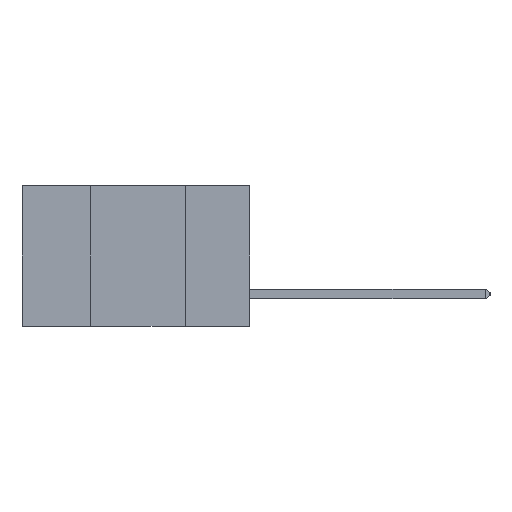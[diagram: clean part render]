
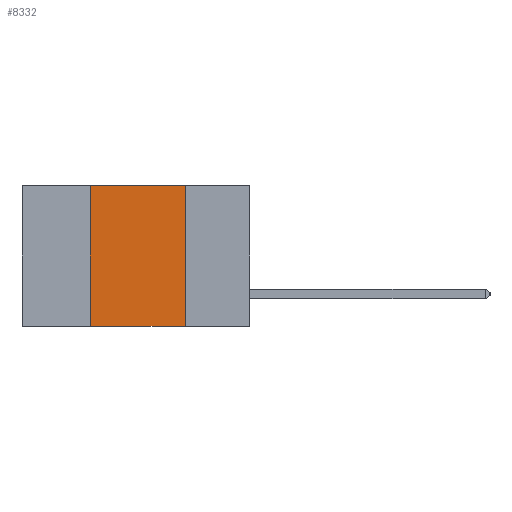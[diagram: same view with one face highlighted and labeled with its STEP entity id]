
A CAD part, left-side view. The second image highlights one B-rep face of the part: STEP entity #8332.
In plain terms, the highlighted planar face has unit normal (-1, 0, 0).
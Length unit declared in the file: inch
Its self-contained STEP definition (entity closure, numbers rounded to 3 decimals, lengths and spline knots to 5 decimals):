
#283 = VERTEX_POINT ( 'NONE', #540 ) ;
#540 = CARTESIAN_POINT ( 'NONE',  ( 0., 0.42, 0. ) ) ;
#607 = PLANE ( 'NONE',  #7331 ) ;
#1368 = ORIENTED_EDGE ( 'NONE', *, *, #8800, .T. ) ;
#1800 = CARTESIAN_POINT ( 'NONE',  ( 0., 0.6, 0. ) ) ;
#1893 = DIRECTION ( 'NONE',  ( 0., 0., 1. ) ) ;
#2639 = VECTOR ( 'NONE', #13578, 39.37008 ) ;
#3047 = LINE ( 'NONE', #1800, #2639 ) ;
#3228 = DIRECTION ( 'NONE',  ( 0., 0., -1. ) ) ;
#3858 = ORIENTED_EDGE ( 'NONE', *, *, #9473, .F. ) ;
#3897 = VECTOR ( 'NONE', #13784, 39.37008 ) ;
#3957 = LINE ( 'NONE', #13613, #10052 ) ;
#4215 = CARTESIAN_POINT ( 'NONE',  ( 0., 0.6, -0.37 ) ) ;
#5959 = CARTESIAN_POINT ( 'NONE',  ( 0., 0.17, 0. ) ) ;
#6720 = ORIENTED_EDGE ( 'NONE', *, *, #10969, .F. ) ;
#6977 = LINE ( 'NONE', #5959, #3897 ) ;
#7331 = AXIS2_PLACEMENT_3D ( 'NONE', #12328, #11041, #3228 ) ;
#7890 = VERTEX_POINT ( 'NONE', #16397 ) ;
#8165 = VERTEX_POINT ( 'NONE', #13302 ) ;
#8332 = ADVANCED_FACE ( 'NONE', ( #14556 ), #607, .F. ) ;
#8403 = CARTESIAN_POINT ( 'NONE',  ( 0., 0.17, -0.37 ) ) ;
#8800 = EDGE_CURVE ( 'NONE', #8165, #16331, #13306, .T. ) ;
#9473 = EDGE_CURVE ( 'NONE', #283, #7890, #3047, .T. ) ;
#9799 = VECTOR ( 'NONE', #10736, 39.37008 ) ;
#10052 = VECTOR ( 'NONE', #1893, 39.37008 ) ;
#10736 = DIRECTION ( 'NONE',  ( 0., -1., 0. ) ) ;
#10969 = EDGE_CURVE ( 'NONE', #8165, #283, #3957, .T. ) ;
#11041 = DIRECTION ( 'NONE',  ( 1., 0., 0. ) ) ;
#11314 = ORIENTED_EDGE ( 'NONE', *, *, #12287, .F. ) ;
#12287 = EDGE_CURVE ( 'NONE', #7890, #16331, #6977, .T. ) ;
#12328 = CARTESIAN_POINT ( 'NONE',  ( 0., 0.6, 0. ) ) ;
#13302 = CARTESIAN_POINT ( 'NONE',  ( 0., 0.42, -0.37 ) ) ;
#13306 = LINE ( 'NONE', #4215, #9799 ) ;
#13578 = DIRECTION ( 'NONE',  ( 0., -1., 0. ) ) ;
#13613 = CARTESIAN_POINT ( 'NONE',  ( 0., 0.42, 0. ) ) ;
#13784 = DIRECTION ( 'NONE',  ( 0., 0., -1. ) ) ;
#13804 = EDGE_LOOP ( 'NONE', ( #11314, #3858, #6720, #1368 ) ) ;
#14556 = FACE_OUTER_BOUND ( 'NONE', #13804, .T. ) ;
#16331 = VERTEX_POINT ( 'NONE', #8403 ) ;
#16397 = CARTESIAN_POINT ( 'NONE',  ( 0., 0.17, 0. ) ) ;
